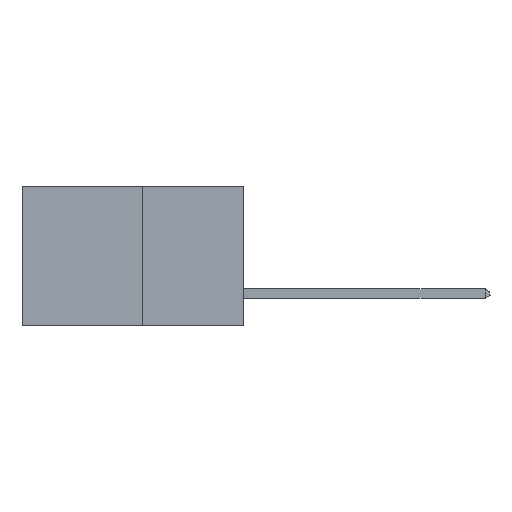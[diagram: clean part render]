
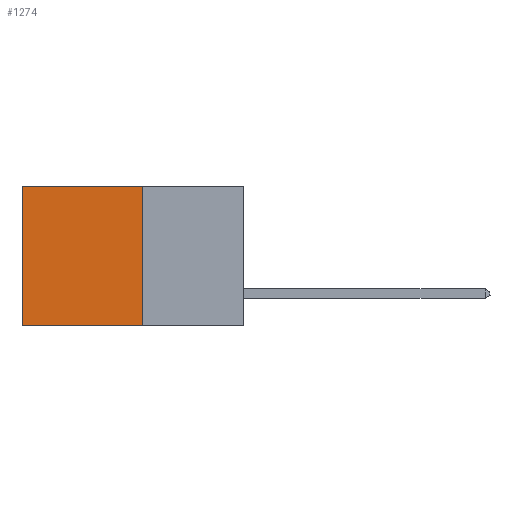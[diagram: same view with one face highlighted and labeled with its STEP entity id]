
A CAD part, left-side view. The second image highlights one B-rep face of the part: STEP entity #1274.
In plain terms, the highlighted planar face has unit normal (-1, 0, 0).
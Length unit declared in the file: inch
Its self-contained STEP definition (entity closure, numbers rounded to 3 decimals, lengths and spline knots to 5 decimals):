
#539 = ORIENTED_EDGE ( 'NONE', *, *, #11992, .F. ) ;
#665 = VECTOR ( 'NONE', #2774, 39.37008 ) ;
#1274 = ADVANCED_FACE ( 'NONE', ( #20125 ), #19384, .F. ) ;
#1388 = VECTOR ( 'NONE', #2458, 39.37008 ) ;
#1491 = LINE ( 'NONE', #10468, #665 ) ;
#2458 = DIRECTION ( 'NONE',  ( 0., 0., -1. ) ) ;
#2774 = DIRECTION ( 'NONE',  ( 0., 1., 0. ) ) ;
#7606 = CARTESIAN_POINT ( 'NONE',  ( 0.277, 0.59, -0.37 ) ) ;
#7668 = VERTEX_POINT ( 'NONE', #28113 ) ;
#7701 = CARTESIAN_POINT ( 'NONE',  ( 0.277, 0.27, 0. ) ) ;
#9130 = LINE ( 'NONE', #14466, #15019 ) ;
#10468 = CARTESIAN_POINT ( 'NONE',  ( 0.277, 0.27, 0. ) ) ;
#10733 = EDGE_CURVE ( 'NONE', #14527, #28417, #1491, .T. ) ;
#11992 = EDGE_CURVE ( 'NONE', #14527, #7668, #20952, .T. ) ;
#12219 = VERTEX_POINT ( 'NONE', #23727 ) ;
#12891 = ORIENTED_EDGE ( 'NONE', *, *, #13912, .T. ) ;
#13912 = EDGE_CURVE ( 'NONE', #28417, #12219, #21763, .T. ) ;
#14466 = CARTESIAN_POINT ( 'NONE',  ( 0.277, 0.27, -0.37 ) ) ;
#14527 = VERTEX_POINT ( 'NONE', #7701 ) ;
#15019 = VECTOR ( 'NONE', #17030, 39.37008 ) ;
#15122 = CARTESIAN_POINT ( 'NONE',  ( 0.277, 0.27, -0.37 ) ) ;
#16549 = VECTOR ( 'NONE', #25408, 39.37008 ) ;
#17030 = DIRECTION ( 'NONE',  ( 0., 1., 0. ) ) ;
#19384 = PLANE ( 'NONE',  #30878 ) ;
#19853 = EDGE_LOOP ( 'NONE', ( #12891, #29889, #539, #28648 ) ) ;
#20125 = FACE_OUTER_BOUND ( 'NONE', #19853, .T. ) ;
#20952 = LINE ( 'NONE', #15122, #1388 ) ;
#21123 = CARTESIAN_POINT ( 'NONE',  ( 0.277, 0.59, 0. ) ) ;
#21763 = LINE ( 'NONE', #7606, #16549 ) ;
#23727 = CARTESIAN_POINT ( 'NONE',  ( 0.277, 0.59, -0.37 ) ) ;
#25408 = DIRECTION ( 'NONE',  ( 0., 0., -1. ) ) ;
#26898 = CARTESIAN_POINT ( 'NONE',  ( 0.277, 0.27, -0.37 ) ) ;
#28113 = CARTESIAN_POINT ( 'NONE',  ( 0.277, 0.27, -0.37 ) ) ;
#28417 = VERTEX_POINT ( 'NONE', #21123 ) ;
#28648 = ORIENTED_EDGE ( 'NONE', *, *, #10733, .T. ) ;
#29889 = ORIENTED_EDGE ( 'NONE', *, *, #31696, .F. ) ;
#30493 = DIRECTION ( 'NONE',  ( 1., 0., 0. ) ) ;
#30878 = AXIS2_PLACEMENT_3D ( 'NONE', #26898, #30493, #31873 ) ;
#31696 = EDGE_CURVE ( 'NONE', #7668, #12219, #9130, .T. ) ;
#31873 = DIRECTION ( 'NONE',  ( 0., 0., -1. ) ) ;
